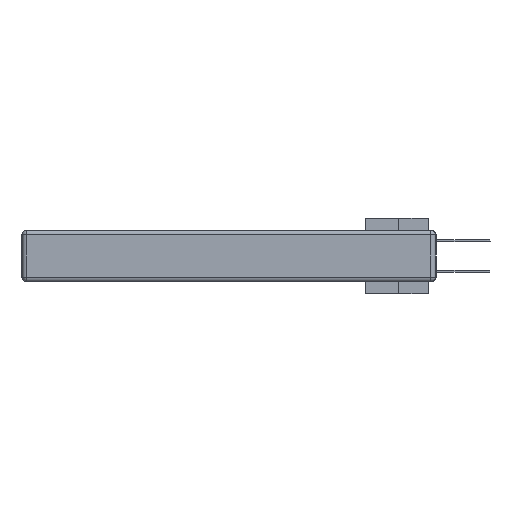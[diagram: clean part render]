
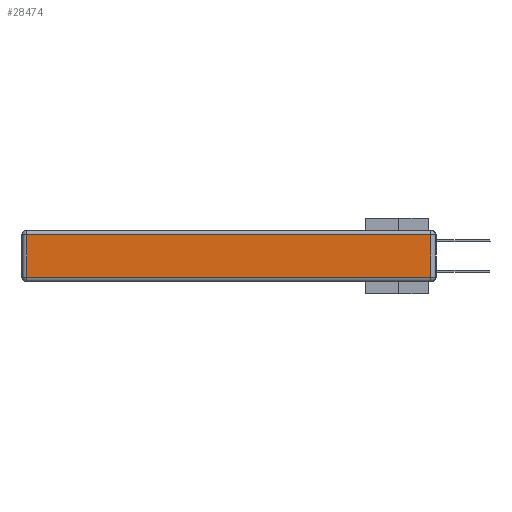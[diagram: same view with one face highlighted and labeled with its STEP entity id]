
A CAD part, left-side view. The second image highlights one B-rep face of the part: STEP entity #28474.
In plain terms, the highlighted planar face has unit normal (-1, 0, 0).
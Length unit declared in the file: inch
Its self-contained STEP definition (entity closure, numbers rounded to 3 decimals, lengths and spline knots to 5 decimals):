
#1805 = CARTESIAN_POINT ( 'NONE',  ( 0., 0., -0.313 ) ) ;
#2519 = CARTESIAN_POINT ( 'NONE',  ( 0., 0.03, -0.313 ) ) ;
#2970 = EDGE_CURVE ( 'NONE', #22858, #24531, #26319, .T. ) ;
#3067 = CARTESIAN_POINT ( 'NONE',  ( 0., 0., -0.343 ) ) ;
#3092 = DIRECTION ( 'NONE',  ( 0., 0., -1. ) ) ;
#3308 = ORIENTED_EDGE ( 'NONE', *, *, #21004, .T. ) ;
#4027 = ORIENTED_EDGE ( 'NONE', *, *, #13361, .T. ) ;
#4783 = EDGE_LOOP ( 'NONE', ( #21026, #7596, #3308, #4027 ) ) ;
#5333 = LINE ( 'NONE', #14391, #7946 ) ;
#6088 = DIRECTION ( 'NONE',  ( 0., 0., 1. ) ) ;
#7596 = ORIENTED_EDGE ( 'NONE', *, *, #2970, .T. ) ;
#7946 = VECTOR ( 'NONE', #3092, 39.37008 ) ;
#9111 = CARTESIAN_POINT ( 'NONE',  ( 0., 2.75, -0.03 ) ) ;
#11018 = DIRECTION ( 'NONE',  ( 0., -1., 0. ) ) ;
#12805 = LINE ( 'NONE', #1805, #15438 ) ;
#13323 = VECTOR ( 'NONE', #6088, 39.37008 ) ;
#13361 = EDGE_CURVE ( 'NONE', #26014, #16331, #5333, .T. ) ;
#14391 = CARTESIAN_POINT ( 'NONE',  ( 0., 2.72, -0.343 ) ) ;
#14995 = EDGE_CURVE ( 'NONE', #16331, #22858, #12805, .T. ) ;
#15269 = CARTESIAN_POINT ( 'NONE',  ( 0., 0.03, -0.03 ) ) ;
#15438 = VECTOR ( 'NONE', #11018, 39.37008 ) ;
#16331 = VERTEX_POINT ( 'NONE', #28476 ) ;
#18513 = PLANE ( 'NONE',  #19263 ) ;
#19263 = AXIS2_PLACEMENT_3D ( 'NONE', #3067, #28055, #27604 ) ;
#21004 = EDGE_CURVE ( 'NONE', #24531, #26014, #24894, .T. ) ;
#21026 = ORIENTED_EDGE ( 'NONE', *, *, #14995, .T. ) ;
#22858 = VERTEX_POINT ( 'NONE', #2519 ) ;
#24531 = VERTEX_POINT ( 'NONE', #15269 ) ;
#24812 = CARTESIAN_POINT ( 'NONE',  ( 0., 2.72, -0.03 ) ) ;
#24894 = LINE ( 'NONE', #9111, #28959 ) ;
#25188 = DIRECTION ( 'NONE',  ( 0., 1., 0. ) ) ;
#25539 = FACE_OUTER_BOUND ( 'NONE', #4783, .T. ) ;
#26014 = VERTEX_POINT ( 'NONE', #24812 ) ;
#26176 = CARTESIAN_POINT ( 'NONE',  ( 0., 0.03, -0.343 ) ) ;
#26319 = LINE ( 'NONE', #26176, #13323 ) ;
#27604 = DIRECTION ( 'NONE',  ( 0., 0., 1. ) ) ;
#28055 = DIRECTION ( 'NONE',  ( -1., 0., 0. ) ) ;
#28474 = ADVANCED_FACE ( 'NONE', ( #25539 ), #18513, .T. ) ;
#28476 = CARTESIAN_POINT ( 'NONE',  ( 0., 2.72, -0.313 ) ) ;
#28959 = VECTOR ( 'NONE', #25188, 39.37008 ) ;
